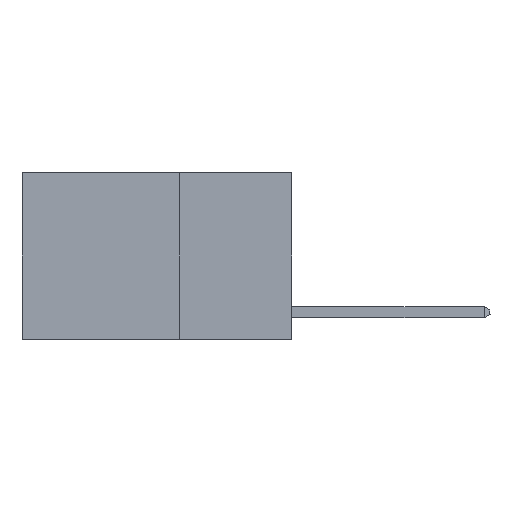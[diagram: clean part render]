
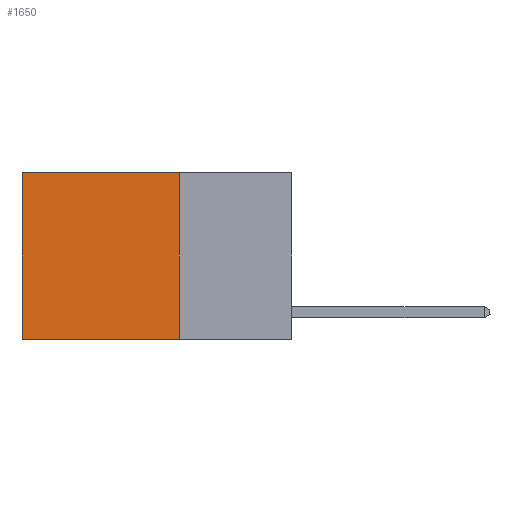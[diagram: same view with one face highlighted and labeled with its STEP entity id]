
A CAD part, left-side view. The second image highlights one B-rep face of the part: STEP entity #1650.
In plain terms, the highlighted planar face has unit normal (-1, 0, 0).
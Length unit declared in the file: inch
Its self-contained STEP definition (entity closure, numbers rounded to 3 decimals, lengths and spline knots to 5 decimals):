
#536 = VECTOR ( 'NONE', #21472, 39.37008 ) ;
#624 = CARTESIAN_POINT ( 'NONE',  ( 0.2625, 0.25, -0.37 ) ) ;
#1050 = VERTEX_POINT ( 'NONE', #21746 ) ;
#1113 = CARTESIAN_POINT ( 'NONE',  ( 0.2625, 0.25, 0. ) ) ;
#1155 = EDGE_LOOP ( 'NONE', ( #13778, #9770, #12726, #3581 ) ) ;
#1650 = ADVANCED_FACE ( 'NONE', ( #12932 ), #10972, .F. ) ;
#2067 = CARTESIAN_POINT ( 'NONE',  ( 0.2625, 0.25, 0. ) ) ;
#3303 = CARTESIAN_POINT ( 'NONE',  ( 0.2625, 0.6, 0. ) ) ;
#3581 = ORIENTED_EDGE ( 'NONE', *, *, #12451, .T. ) ;
#4353 = AXIS2_PLACEMENT_3D ( 'NONE', #5300, #24904, #21359 ) ;
#5300 = CARTESIAN_POINT ( 'NONE',  ( 0.2625, 0.25, 0. ) ) ;
#6330 = CARTESIAN_POINT ( 'NONE',  ( 0.2625, 0.6, 0. ) ) ;
#8730 = DIRECTION ( 'NONE',  ( 0., 1., 0. ) ) ;
#9735 = EDGE_CURVE ( 'NONE', #1050, #23987, #14067, .T. ) ;
#9770 = ORIENTED_EDGE ( 'NONE', *, *, #25235, .F. ) ;
#10068 = VECTOR ( 'NONE', #8730, 39.37008 ) ;
#10972 = PLANE ( 'NONE',  #4353 ) ;
#11522 = VECTOR ( 'NONE', #14584, 39.37008 ) ;
#12451 = EDGE_CURVE ( 'NONE', #1050, #22007, #21245, .T. ) ;
#12726 = ORIENTED_EDGE ( 'NONE', *, *, #9735, .F. ) ;
#12932 = FACE_OUTER_BOUND ( 'NONE', #1155, .T. ) ;
#13431 = LINE ( 'NONE', #3303, #536 ) ;
#13778 = ORIENTED_EDGE ( 'NONE', *, *, #18761, .T. ) ;
#14067 = LINE ( 'NONE', #2067, #11522 ) ;
#14584 = DIRECTION ( 'NONE',  ( 0., 0., -1. ) ) ;
#16240 = VECTOR ( 'NONE', #25580, 39.37008 ) ;
#16776 = CARTESIAN_POINT ( 'NONE',  ( 0.2625, 0.6, -0.37 ) ) ;
#17357 = VERTEX_POINT ( 'NONE', #16776 ) ;
#18646 = LINE ( 'NONE', #624, #10068 ) ;
#18761 = EDGE_CURVE ( 'NONE', #22007, #17357, #13431, .T. ) ;
#21245 = LINE ( 'NONE', #1113, #16240 ) ;
#21359 = DIRECTION ( 'NONE',  ( 0., 0., -1. ) ) ;
#21472 = DIRECTION ( 'NONE',  ( 0., 0., -1. ) ) ;
#21746 = CARTESIAN_POINT ( 'NONE',  ( 0.2625, 0.25, 0. ) ) ;
#22007 = VERTEX_POINT ( 'NONE', #6330 ) ;
#23987 = VERTEX_POINT ( 'NONE', #25507 ) ;
#24904 = DIRECTION ( 'NONE',  ( 1., 0., 0. ) ) ;
#25235 = EDGE_CURVE ( 'NONE', #23987, #17357, #18646, .T. ) ;
#25507 = CARTESIAN_POINT ( 'NONE',  ( 0.2625, 0.25, -0.37 ) ) ;
#25580 = DIRECTION ( 'NONE',  ( 0., 1., 0. ) ) ;
